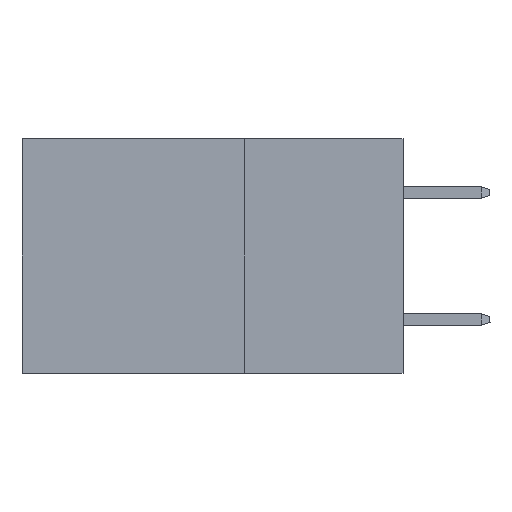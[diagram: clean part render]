
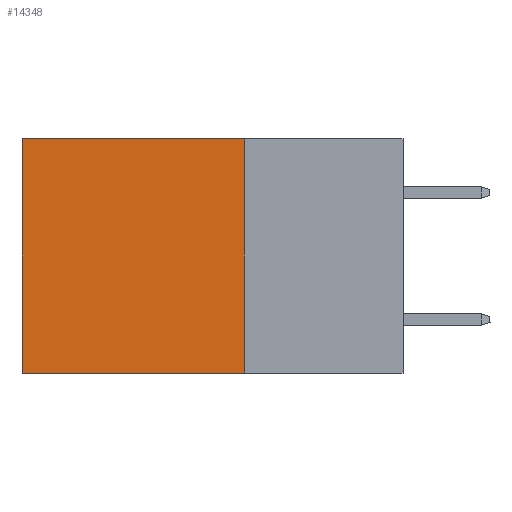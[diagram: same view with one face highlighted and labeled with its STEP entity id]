
A CAD part, left-side view. The second image highlights one B-rep face of the part: STEP entity #14348.
In plain terms, the highlighted planar face has unit normal (-1, 0, 0).
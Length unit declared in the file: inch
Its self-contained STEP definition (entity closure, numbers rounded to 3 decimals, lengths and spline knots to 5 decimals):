
#18 = DIRECTION ( 'NONE',  ( 0., 1., 0. ) ) ;
#325 = DIRECTION ( 'NONE',  ( 0., 1., 0. ) ) ;
#1202 = CARTESIAN_POINT ( 'NONE',  ( 0.2875, 0.25, -0.37 ) ) ;
#2329 = PLANE ( 'NONE',  #14777 ) ;
#3083 = EDGE_LOOP ( 'NONE', ( #7769, #8200, #4719, #6385 ) ) ;
#3624 = EDGE_CURVE ( 'NONE', #7299, #7677, #5141, .T. ) ;
#3937 = CARTESIAN_POINT ( 'NONE',  ( 0.2875, 0.6, 0. ) ) ;
#4050 = CARTESIAN_POINT ( 'NONE',  ( 0.2875, 0.25, 0. ) ) ;
#4345 = FACE_OUTER_BOUND ( 'NONE', #3083, .T. ) ;
#4585 = DIRECTION ( 'NONE',  ( 0., 0., -1. ) ) ;
#4719 = ORIENTED_EDGE ( 'NONE', *, *, #10418, .F. ) ;
#5141 = LINE ( 'NONE', #13260, #14284 ) ;
#5920 = CARTESIAN_POINT ( 'NONE',  ( 0.2875, 0.25, 0. ) ) ;
#6160 = EDGE_CURVE ( 'NONE', #11198, #7677, #7099, .T. ) ;
#6177 = VECTOR ( 'NONE', #18, 39.37008 ) ;
#6385 = ORIENTED_EDGE ( 'NONE', *, *, #13435, .T. ) ;
#7058 = LINE ( 'NONE', #5920, #12673 ) ;
#7099 = LINE ( 'NONE', #1202, #6177 ) ;
#7299 = VERTEX_POINT ( 'NONE', #3937 ) ;
#7358 = CARTESIAN_POINT ( 'NONE',  ( 0.2875, 0.6, -0.37 ) ) ;
#7486 = CARTESIAN_POINT ( 'NONE',  ( 0.2875, 0.25, -0.37 ) ) ;
#7677 = VERTEX_POINT ( 'NONE', #7358 ) ;
#7769 = ORIENTED_EDGE ( 'NONE', *, *, #3624, .T. ) ;
#8200 = ORIENTED_EDGE ( 'NONE', *, *, #6160, .F. ) ;
#9083 = CARTESIAN_POINT ( 'NONE',  ( 0.2875, 0.25, 0. ) ) ;
#9875 = DIRECTION ( 'NONE',  ( 0., 0., -1. ) ) ;
#10418 = EDGE_CURVE ( 'NONE', #12841, #11198, #7058, .T. ) ;
#10550 = VECTOR ( 'NONE', #325, 39.37008 ) ;
#11198 = VERTEX_POINT ( 'NONE', #7486 ) ;
#12673 = VECTOR ( 'NONE', #15386, 39.37008 ) ;
#12841 = VERTEX_POINT ( 'NONE', #4050 ) ;
#13260 = CARTESIAN_POINT ( 'NONE',  ( 0.2875, 0.6, 0. ) ) ;
#13304 = CARTESIAN_POINT ( 'NONE',  ( 0.2875, 0.25, 0. ) ) ;
#13435 = EDGE_CURVE ( 'NONE', #12841, #7299, #14404, .T. ) ;
#14284 = VECTOR ( 'NONE', #9875, 39.37008 ) ;
#14348 = ADVANCED_FACE ( 'NONE', ( #4345 ), #2329, .F. ) ;
#14404 = LINE ( 'NONE', #13304, #10550 ) ;
#14777 = AXIS2_PLACEMENT_3D ( 'NONE', #9083, #15194, #4585 ) ;
#15194 = DIRECTION ( 'NONE',  ( 1., 0., 0. ) ) ;
#15386 = DIRECTION ( 'NONE',  ( 0., 0., -1. ) ) ;
